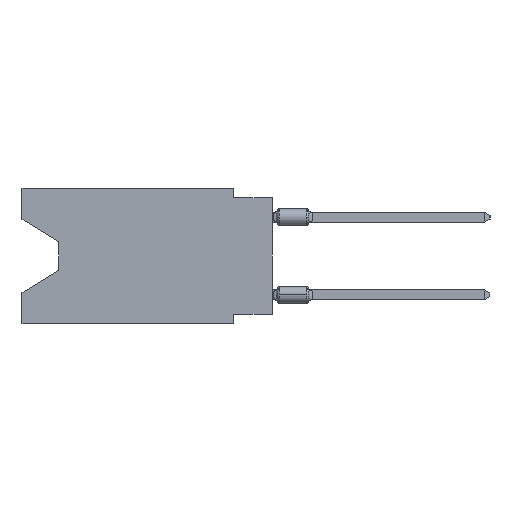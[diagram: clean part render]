
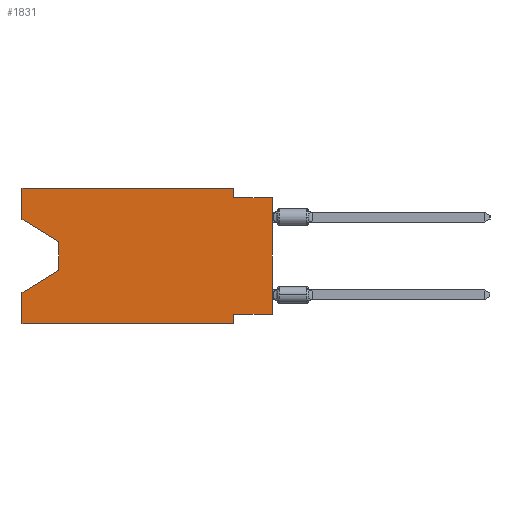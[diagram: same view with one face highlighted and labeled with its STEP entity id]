
A CAD part, left-side view. The second image highlights one B-rep face of the part: STEP entity #1831.
In plain terms, the highlighted planar face has unit normal (-1, 0, 0).
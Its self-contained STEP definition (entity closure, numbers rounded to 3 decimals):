
#807 = DIRECTION ( 'NONE',  ( 0., 0., -1. ) ) ;
#1831 = ADVANCED_FACE ( 'NONE', ( #65658 ), #13558, .F. ) ;
#2499 = VERTEX_POINT ( 'NONE', #2648 ) ;
#2648 = CARTESIAN_POINT ( 'NONE',  ( 0., 16.383, -6.852 ) ) ;
#3276 = LINE ( 'NONE', #39062, #52996 ) ;
#4143 = DIRECTION ( 'NONE',  ( 0., 0., 1. ) ) ;
#4376 = LINE ( 'NONE', #8822, #29531 ) ;
#6507 = VERTEX_POINT ( 'NONE', #50236 ) ;
#6715 = DIRECTION ( 'NONE',  ( 0., 0.855, -0.519 ) ) ;
#6913 = CARTESIAN_POINT ( 'NONE',  ( 0., 16.383, 0. ) ) ;
#7564 = CARTESIAN_POINT ( 'NONE',  ( 0., 13.97, -3.505 ) ) ;
#8334 = EDGE_CURVE ( 'NONE', #17658, #33582, #51148, .T. ) ;
#8580 = EDGE_CURVE ( 'NONE', #6507, #2499, #49057, .T. ) ;
#8621 = CARTESIAN_POINT ( 'NONE',  ( 0., 13.97, -3.505 ) ) ;
#8822 = CARTESIAN_POINT ( 'NONE',  ( 0., 16.383, -2.038 ) ) ;
#9081 = ORIENTED_EDGE ( 'NONE', *, *, #47063, .T. ) ;
#9106 = EDGE_CURVE ( 'NONE', #44358, #30752, #15143, .T. ) ;
#11317 = ORIENTED_EDGE ( 'NONE', *, *, #63821, .F. ) ;
#12362 = CARTESIAN_POINT ( 'NONE',  ( 0., 0., -0.635 ) ) ;
#12885 = DIRECTION ( 'NONE',  ( 0., 0., -1. ) ) ;
#13558 = PLANE ( 'NONE',  #41209 ) ;
#14949 = EDGE_CURVE ( 'NONE', #19078, #56506, #3276, .T. ) ;
#15143 = LINE ( 'NONE', #36584, #29801 ) ;
#15205 = CARTESIAN_POINT ( 'NONE',  ( 0., 0., -8.255 ) ) ;
#15735 = CARTESIAN_POINT ( 'NONE',  ( 0., 2.54, -8.89 ) ) ;
#15924 = VECTOR ( 'NONE', #30921, 1000. ) ;
#17423 = VECTOR ( 'NONE', #44586, 1000. ) ;
#17658 = VERTEX_POINT ( 'NONE', #32468 ) ;
#18360 = EDGE_LOOP ( 'NONE', ( #51878, #62948, #9081, #27021, #24205, #40900, #21901, #48339, #11317, #53801, #20134, #38321 ) ) ;
#19078 = VERTEX_POINT ( 'NONE', #6913 ) ;
#19613 = EDGE_CURVE ( 'NONE', #35203, #36930, #4376, .T. ) ;
#20134 = ORIENTED_EDGE ( 'NONE', *, *, #14949, .F. ) ;
#21279 = CARTESIAN_POINT ( 'NONE',  ( 0., 2.54, 0. ) ) ;
#21727 = EDGE_CURVE ( 'NONE', #35203, #19078, #62959, .T. ) ;
#21901 = ORIENTED_EDGE ( 'NONE', *, *, #29931, .F. ) ;
#22278 = VECTOR ( 'NONE', #6715, 1000. ) ;
#23812 = LINE ( 'NONE', #27926, #17423 ) ;
#24205 = ORIENTED_EDGE ( 'NONE', *, *, #65482, .T. ) ;
#27021 = ORIENTED_EDGE ( 'NONE', *, *, #8580, .F. ) ;
#27926 = CARTESIAN_POINT ( 'NONE',  ( 0., 16.383, -8.89 ) ) ;
#29531 = VECTOR ( 'NONE', #29612, 1000. ) ;
#29607 = CARTESIAN_POINT ( 'NONE',  ( 0., 16.383, -2.038 ) ) ;
#29612 = DIRECTION ( 'NONE',  ( 0., -0.855, -0.519 ) ) ;
#29801 = VECTOR ( 'NONE', #807, 1000. ) ;
#29931 = EDGE_CURVE ( 'NONE', #17658, #44358, #61862, .T. ) ;
#30752 = VERTEX_POINT ( 'NONE', #15735 ) ;
#30921 = DIRECTION ( 'NONE',  ( 0., -1., 0. ) ) ;
#32468 = CARTESIAN_POINT ( 'NONE',  ( 0., 0., -8.255 ) ) ;
#33582 = VERTEX_POINT ( 'NONE', #12362 ) ;
#33649 = VECTOR ( 'NONE', #35545, 1000. ) ;
#34336 = CARTESIAN_POINT ( 'NONE',  ( 0., 16.383, 0. ) ) ;
#34938 = VECTOR ( 'NONE', #62536, 1000. ) ;
#35203 = VERTEX_POINT ( 'NONE', #29607 ) ;
#35545 = DIRECTION ( 'NONE',  ( 0., 0., -1. ) ) ;
#36584 = CARTESIAN_POINT ( 'NONE',  ( 0., 2.54, -8.89 ) ) ;
#36930 = VERTEX_POINT ( 'NONE', #7564 ) ;
#37276 = VERTEX_POINT ( 'NONE', #63706 ) ;
#38321 = ORIENTED_EDGE ( 'NONE', *, *, #21727, .F. ) ;
#38851 = DIRECTION ( 'NONE',  ( 0., 0., 1. ) ) ;
#39062 = CARTESIAN_POINT ( 'NONE',  ( 0., 16.383, 0. ) ) ;
#40443 = VECTOR ( 'NONE', #38851, 1000. ) ;
#40900 = ORIENTED_EDGE ( 'NONE', *, *, #9106, .F. ) ;
#41209 = AXIS2_PLACEMENT_3D ( 'NONE', #34336, #49664, #12885 ) ;
#42183 = CARTESIAN_POINT ( 'NONE',  ( 0., 16.383, 0. ) ) ;
#42514 = DIRECTION ( 'NONE',  ( 0., 0., 1. ) ) ;
#44358 = VERTEX_POINT ( 'NONE', #45563 ) ;
#44586 = DIRECTION ( 'NONE',  ( 0., -1., 0. ) ) ;
#45329 = CARTESIAN_POINT ( 'NONE',  ( 0., 2.54, 0. ) ) ;
#45563 = CARTESIAN_POINT ( 'NONE',  ( 0., 2.54, -8.255 ) ) ;
#46979 = VECTOR ( 'NONE', #42514, 1000. ) ;
#47063 = EDGE_CURVE ( 'NONE', #47427, #2499, #59176, .T. ) ;
#47427 = VERTEX_POINT ( 'NONE', #53321 ) ;
#48339 = ORIENTED_EDGE ( 'NONE', *, *, #8334, .T. ) ;
#49057 = LINE ( 'NONE', #55500, #40443 ) ;
#49664 = DIRECTION ( 'NONE',  ( 1., 0., 0. ) ) ;
#49851 = VECTOR ( 'NONE', #60988, 1000. ) ;
#50236 = CARTESIAN_POINT ( 'NONE',  ( 0., 16.383, -8.89 ) ) ;
#51148 = LINE ( 'NONE', #61703, #64338 ) ;
#51368 = LINE ( 'NONE', #56126, #15924 ) ;
#51878 = ORIENTED_EDGE ( 'NONE', *, *, #19613, .T. ) ;
#52075 = EDGE_CURVE ( 'NONE', #56506, #37276, #59991, .T. ) ;
#52855 = EDGE_CURVE ( 'NONE', #36930, #47427, #55315, .T. ) ;
#52996 = VECTOR ( 'NONE', #65621, 1000. ) ;
#53321 = CARTESIAN_POINT ( 'NONE',  ( 0., 13.97, -5.385 ) ) ;
#53395 = CARTESIAN_POINT ( 'NONE',  ( 0., 13.97, -5.385 ) ) ;
#53801 = ORIENTED_EDGE ( 'NONE', *, *, #52075, .F. ) ;
#55315 = LINE ( 'NONE', #8621, #33649 ) ;
#55500 = CARTESIAN_POINT ( 'NONE',  ( 0., 16.383, 0. ) ) ;
#56126 = CARTESIAN_POINT ( 'NONE',  ( 0., 0., -0.635 ) ) ;
#56506 = VERTEX_POINT ( 'NONE', #21279 ) ;
#59176 = LINE ( 'NONE', #53395, #22278 ) ;
#59991 = LINE ( 'NONE', #45329, #49851 ) ;
#60988 = DIRECTION ( 'NONE',  ( 0., 0., -1. ) ) ;
#61703 = CARTESIAN_POINT ( 'NONE',  ( 0., 0., 0. ) ) ;
#61862 = LINE ( 'NONE', #15205, #34938 ) ;
#62536 = DIRECTION ( 'NONE',  ( 0., 1., 0. ) ) ;
#62948 = ORIENTED_EDGE ( 'NONE', *, *, #52855, .T. ) ;
#62959 = LINE ( 'NONE', #42183, #46979 ) ;
#63706 = CARTESIAN_POINT ( 'NONE',  ( 0., 2.54, -0.635 ) ) ;
#63821 = EDGE_CURVE ( 'NONE', #37276, #33582, #51368, .T. ) ;
#64338 = VECTOR ( 'NONE', #4143, 1000. ) ;
#65482 = EDGE_CURVE ( 'NONE', #6507, #30752, #23812, .T. ) ;
#65621 = DIRECTION ( 'NONE',  ( 0., -1., 0. ) ) ;
#65658 = FACE_OUTER_BOUND ( 'NONE', #18360, .T. ) ;
